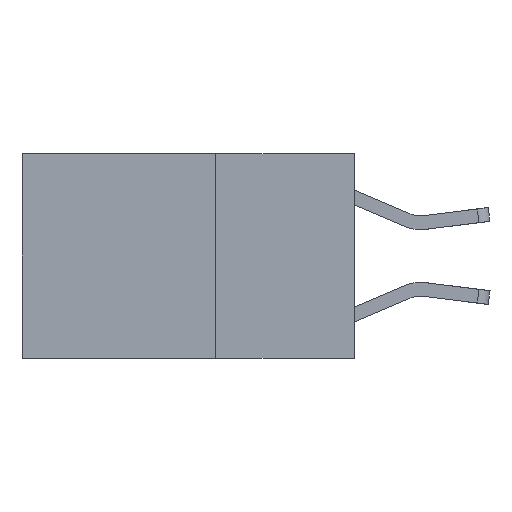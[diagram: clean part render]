
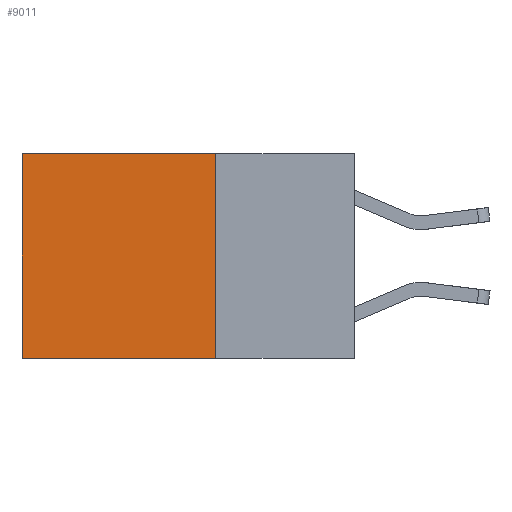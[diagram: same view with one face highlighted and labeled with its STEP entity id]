
A CAD part, left-side view. The second image highlights one B-rep face of the part: STEP entity #9011.
In plain terms, the highlighted planar face has unit normal (-1, 0, 0).
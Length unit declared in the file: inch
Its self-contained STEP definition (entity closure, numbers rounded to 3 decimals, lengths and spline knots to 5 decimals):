
#120 = VERTEX_POINT ( 'NONE', #2641 ) ;
#575 = VERTEX_POINT ( 'NONE', #12297 ) ;
#716 = CARTESIAN_POINT ( 'NONE',  ( 0.2625, 0.25, 0. ) ) ;
#778 = EDGE_LOOP ( 'NONE', ( #5123, #5642, #5948, #8050 ) ) ;
#868 = CARTESIAN_POINT ( 'NONE',  ( 0.2625, 0.25, 0. ) ) ;
#965 = CARTESIAN_POINT ( 'NONE',  ( 0.2625, 0.6, -0.37 ) ) ;
#1777 = CARTESIAN_POINT ( 'NONE',  ( 0.2625, 0.25, -0.37 ) ) ;
#1894 = EDGE_CURVE ( 'NONE', #120, #575, #9335, .T. ) ;
#2212 = CARTESIAN_POINT ( 'NONE',  ( 0.2625, 0.25, 0. ) ) ;
#2641 = CARTESIAN_POINT ( 'NONE',  ( 0.2625, 0.25, 0. ) ) ;
#2978 = VECTOR ( 'NONE', #5524, 39.37008 ) ;
#4152 = DIRECTION ( 'NONE',  ( 0., 0., -1. ) ) ;
#4938 = LINE ( 'NONE', #868, #2978 ) ;
#5088 = VERTEX_POINT ( 'NONE', #5828 ) ;
#5123 = ORIENTED_EDGE ( 'NONE', *, *, #6147, .T. ) ;
#5524 = DIRECTION ( 'NONE',  ( 0., 1., 0. ) ) ;
#5642 = ORIENTED_EDGE ( 'NONE', *, *, #10586, .F. ) ;
#5783 = VECTOR ( 'NONE', #6538, 39.37008 ) ;
#5828 = CARTESIAN_POINT ( 'NONE',  ( 0.2625, 0.6, 0. ) ) ;
#5948 = ORIENTED_EDGE ( 'NONE', *, *, #1894, .F. ) ;
#6147 = EDGE_CURVE ( 'NONE', #5088, #9454, #6240, .T. ) ;
#6240 = LINE ( 'NONE', #8937, #6693 ) ;
#6538 = DIRECTION ( 'NONE',  ( 0., 0., -1. ) ) ;
#6669 = AXIS2_PLACEMENT_3D ( 'NONE', #2212, #8018, #4152 ) ;
#6693 = VECTOR ( 'NONE', #7937, 39.37008 ) ;
#7306 = VECTOR ( 'NONE', #8443, 39.37008 ) ;
#7934 = PLANE ( 'NONE',  #6669 ) ;
#7937 = DIRECTION ( 'NONE',  ( 0., 0., -1. ) ) ;
#8018 = DIRECTION ( 'NONE',  ( 1., 0., 0. ) ) ;
#8050 = ORIENTED_EDGE ( 'NONE', *, *, #9948, .T. ) ;
#8443 = DIRECTION ( 'NONE',  ( 0., 1., 0. ) ) ;
#8937 = CARTESIAN_POINT ( 'NONE',  ( 0.2625, 0.6, 0. ) ) ;
#9011 = ADVANCED_FACE ( 'NONE', ( #11384 ), #7934, .F. ) ;
#9335 = LINE ( 'NONE', #716, #5783 ) ;
#9454 = VERTEX_POINT ( 'NONE', #965 ) ;
#9835 = LINE ( 'NONE', #1777, #7306 ) ;
#9948 = EDGE_CURVE ( 'NONE', #120, #5088, #4938, .T. ) ;
#10586 = EDGE_CURVE ( 'NONE', #575, #9454, #9835, .T. ) ;
#11384 = FACE_OUTER_BOUND ( 'NONE', #778, .T. ) ;
#12297 = CARTESIAN_POINT ( 'NONE',  ( 0.2625, 0.25, -0.37 ) ) ;
